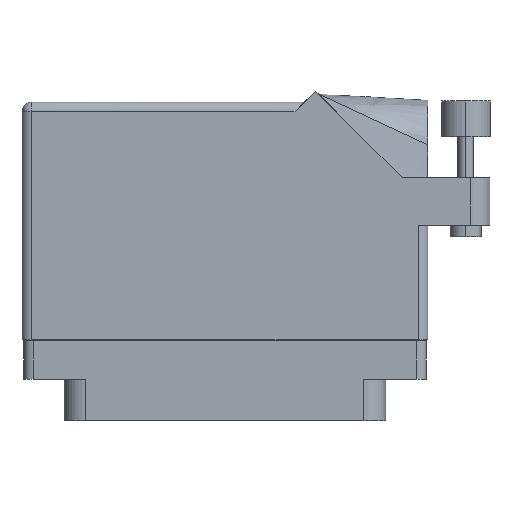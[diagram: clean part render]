
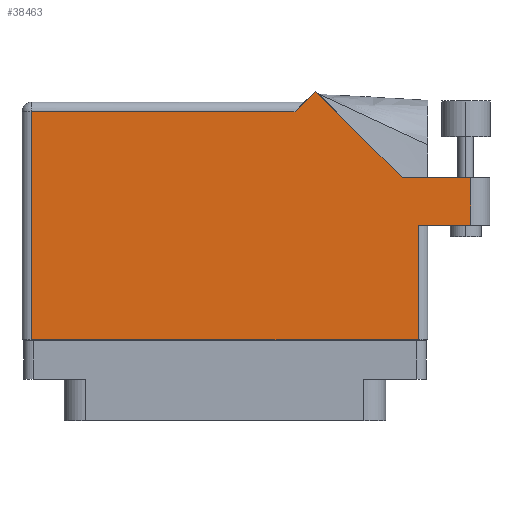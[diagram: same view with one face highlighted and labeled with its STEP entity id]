
A CAD part, front view. The second image highlights one B-rep face of the part: STEP entity #38463.
In plain terms, the highlighted face is planar.
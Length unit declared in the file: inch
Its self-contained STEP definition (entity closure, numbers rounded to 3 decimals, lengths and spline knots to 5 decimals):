
#18 = LINE ( 'NONE', #27056, #43236 ) ;
#256 = LINE ( 'NONE', #12790, #50373 ) ;
#536 = DIRECTION ( 'NONE',  ( -1., 0., 0. ) ) ;
#942 = VECTOR ( 'NONE', #2680, 39.37008 ) ;
#1663 = PLANE ( 'NONE',  #48317 ) ;
#2680 = DIRECTION ( 'NONE',  ( 0., 1., 0. ) ) ;
#3174 = LINE ( 'NONE', #24442, #37705 ) ;
#4926 = ORIENTED_EDGE ( 'NONE', *, *, #9631, .T. ) ;
#6267 = CARTESIAN_POINT ( 'NONE',  ( 1.306, 0.637, 0.455 ) ) ;
#6370 = CARTESIAN_POINT ( 'NONE',  ( 1.706, 0.944, 0.455 ) ) ;
#6922 = DIRECTION ( 'NONE',  ( -1., 0., 0. ) ) ;
#8162 = LINE ( 'NONE', #51297, #49519 ) ;
#9631 = EDGE_CURVE ( 'NONE', #15773, #48675, #29721, .T. ) ;
#9744 = CARTESIAN_POINT ( 'NONE',  ( -1.306, 1.43, 0.455 ) ) ;
#10319 = DIRECTION ( 'NONE',  ( 1., 0., 0. ) ) ;
#12527 = EDGE_CURVE ( 'NONE', #44699, #30081, #42222, .T. ) ;
#12790 = CARTESIAN_POINT ( 'NONE',  ( -1.306, 1.368, 0.455 ) ) ;
#13291 = VERTEX_POINT ( 'NONE', #47778 ) ;
#15173 = CARTESIAN_POINT ( 'NONE',  ( -1.244, -0.1, 0.455 ) ) ;
#15773 = VERTEX_POINT ( 'NONE', #41525 ) ;
#17284 = EDGE_CURVE ( 'NONE', #40199, #48620, #21874, .T. ) ;
#18786 = ORIENTED_EDGE ( 'NONE', *, *, #17284, .T. ) ;
#19364 = DIRECTION ( 'NONE',  ( 0., -1., 0. ) ) ;
#20018 = FACE_OUTER_BOUND ( 'NONE', #39868, .T. ) ;
#20133 = VERTEX_POINT ( 'NONE', #21690 ) ;
#21044 = EDGE_CURVE ( 'NONE', #30081, #20133, #8162, .T. ) ;
#21430 = EDGE_CURVE ( 'NONE', #20133, #27288, #18, .T. ) ;
#21690 = CARTESIAN_POINT ( 'NONE',  ( 0.58371, 1.50071, 0.455 ) ) ;
#21874 = LINE ( 'NONE', #50259, #25032 ) ;
#22196 = VECTOR ( 'NONE', #10319, 39.37008 ) ;
#22389 = CARTESIAN_POINT ( 'NONE',  ( 1.581, 0.944, 0.455 ) ) ;
#22503 = CARTESIAN_POINT ( 'NONE',  ( 1.244, -0.1, 0.455 ) ) ;
#22771 = ORIENTED_EDGE ( 'NONE', *, *, #29309, .T. ) ;
#24008 = ORIENTED_EDGE ( 'NONE', *, *, #21430, .T. ) ;
#24442 = CARTESIAN_POINT ( 'NONE',  ( 1.244, 0.637, 0.455 ) ) ;
#25032 = VECTOR ( 'NONE', #50444, 39.37008 ) ;
#25834 = DIRECTION ( 'NONE',  ( 0., 0., -1. ) ) ;
#25877 = EDGE_CURVE ( 'NONE', #48620, #15773, #3174, .T. ) ;
#26522 = CARTESIAN_POINT ( 'NONE',  ( 1.581, 0.637, 0.455 ) ) ;
#27056 = CARTESIAN_POINT ( 'NONE',  ( 0.513, 1.43, 0.455 ) ) ;
#27288 = VERTEX_POINT ( 'NONE', #49807 ) ;
#29309 = EDGE_CURVE ( 'NONE', #27288, #13291, #256, .T. ) ;
#29692 = CARTESIAN_POINT ( 'NONE',  ( -1.244, -0.1, 0.455 ) ) ;
#29721 = LINE ( 'NONE', #6267, #22196 ) ;
#30081 = VERTEX_POINT ( 'NONE', #42383 ) ;
#30729 = DIRECTION ( 'NONE',  ( -0.707, -0.707, 0. ) ) ;
#30925 = ORIENTED_EDGE ( 'NONE', *, *, #48585, .T. ) ;
#34634 = DIRECTION ( 'NONE',  ( -1., 0., 0. ) ) ;
#35482 = LINE ( 'NONE', #50677, #942 ) ;
#36487 = ORIENTED_EDGE ( 'NONE', *, *, #21044, .T. ) ;
#37705 = VECTOR ( 'NONE', #51789, 39.37008 ) ;
#38463 = ADVANCED_FACE ( 'NONE', ( #20018 ), #1663, .F. ) ;
#39868 = EDGE_LOOP ( 'NONE', ( #4926, #30925, #50115, #36487, #24008, #22771, #42280, #18786, #49164 ) ) ;
#40199 = VERTEX_POINT ( 'NONE', #29692 ) ;
#41525 = CARTESIAN_POINT ( 'NONE',  ( 1.244, 0.637, 0.455 ) ) ;
#42222 = LINE ( 'NONE', #6370, #49757 ) ;
#42280 = ORIENTED_EDGE ( 'NONE', *, *, #49714, .T. ) ;
#42383 = CARTESIAN_POINT ( 'NONE',  ( 1.14042, 0.944, 0.455 ) ) ;
#43236 = VECTOR ( 'NONE', #30729, 39.37008 ) ;
#44699 = VERTEX_POINT ( 'NONE', #22389 ) ;
#47737 = DIRECTION ( 'NONE',  ( -0.707, 0.707, 0. ) ) ;
#47778 = CARTESIAN_POINT ( 'NONE',  ( -1.244, 1.368, 0.455 ) ) ;
#48317 = AXIS2_PLACEMENT_3D ( 'NONE', #9744, #25834, #6922 ) ;
#48585 = EDGE_CURVE ( 'NONE', #48675, #44699, #35482, .T. ) ;
#48620 = VERTEX_POINT ( 'NONE', #22503 ) ;
#48675 = VERTEX_POINT ( 'NONE', #26522 ) ;
#49151 = VECTOR ( 'NONE', #19364, 39.37008 ) ;
#49164 = ORIENTED_EDGE ( 'NONE', *, *, #25877, .T. ) ;
#49519 = VECTOR ( 'NONE', #47737, 39.37008 ) ;
#49714 = EDGE_CURVE ( 'NONE', #13291, #40199, #49749, .T. ) ;
#49749 = LINE ( 'NONE', #15173, #49151 ) ;
#49757 = VECTOR ( 'NONE', #34634, 39.37008 ) ;
#49807 = CARTESIAN_POINT ( 'NONE',  ( 0.451, 1.368, 0.455 ) ) ;
#50115 = ORIENTED_EDGE ( 'NONE', *, *, #12527, .T. ) ;
#50259 = CARTESIAN_POINT ( 'NONE',  ( -1.306, -0.1, 0.455 ) ) ;
#50373 = VECTOR ( 'NONE', #536, 39.37008 ) ;
#50444 = DIRECTION ( 'NONE',  ( 1., 0., 0. ) ) ;
#50677 = CARTESIAN_POINT ( 'NONE',  ( 1.581, 0.944, 0.455 ) ) ;
#51297 = CARTESIAN_POINT ( 'NONE',  ( 1.14042, 0.944, 0.455 ) ) ;
#51789 = DIRECTION ( 'NONE',  ( 0., 1., 0. ) ) ;
